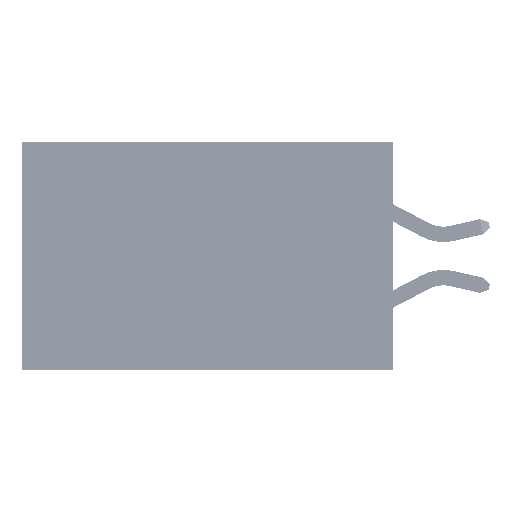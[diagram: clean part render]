
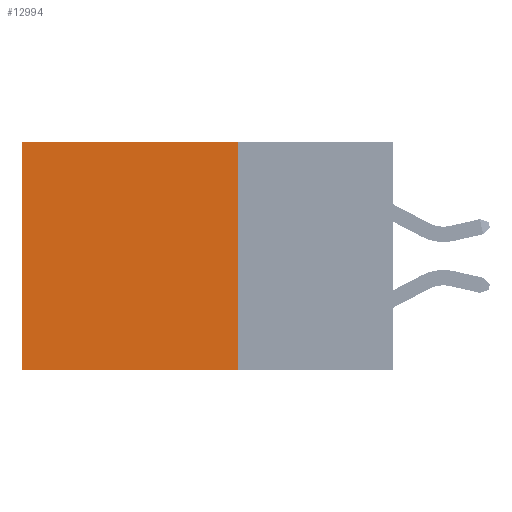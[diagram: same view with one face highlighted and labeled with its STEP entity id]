
A CAD part, left-side view. The second image highlights one B-rep face of the part: STEP entity #12994.
In plain terms, the highlighted planar face has unit normal (-1, 0, 0).
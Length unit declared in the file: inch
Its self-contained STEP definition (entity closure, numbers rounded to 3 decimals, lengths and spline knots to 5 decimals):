
#350 = DIRECTION ( 'NONE',  ( 0., 1., 0. ) ) ;
#1500 = DIRECTION ( 'NONE',  ( 0., 0., -1. ) ) ;
#3335 = ORIENTED_EDGE ( 'NONE', *, *, #19164, .F. ) ;
#4283 = LINE ( 'NONE', #19278, #27918 ) ;
#7785 = CARTESIAN_POINT ( 'NONE',  ( 0.2875, 0.6, -0.37 ) ) ;
#9209 = CARTESIAN_POINT ( 'NONE',  ( 0.2875, 0.25, 0. ) ) ;
#9853 = DIRECTION ( 'NONE',  ( 1., 0., 0. ) ) ;
#11382 = EDGE_LOOP ( 'NONE', ( #16281, #30564, #3335, #38147 ) ) ;
#12994 = ADVANCED_FACE ( 'NONE', ( #17235 ), #32239, .F. ) ;
#13551 = DIRECTION ( 'NONE',  ( 0., 0., -1. ) ) ;
#13638 = LINE ( 'NONE', #9209, #31500 ) ;
#15596 = VERTEX_POINT ( 'NONE', #26380 ) ;
#16281 = ORIENTED_EDGE ( 'NONE', *, *, #23016, .T. ) ;
#17235 = FACE_OUTER_BOUND ( 'NONE', #11382, .T. ) ;
#19063 = DIRECTION ( 'NONE',  ( 0., 0., -1. ) ) ;
#19164 = EDGE_CURVE ( 'NONE', #39890, #15596, #46018, .T. ) ;
#19278 = CARTESIAN_POINT ( 'NONE',  ( 0.2875, 0.25, -0.37 ) ) ;
#23016 = EDGE_CURVE ( 'NONE', #41914, #44384, #45142, .T. ) ;
#24217 = DIRECTION ( 'NONE',  ( 0., 1., 0. ) ) ;
#26380 = CARTESIAN_POINT ( 'NONE',  ( 0.2875, 0.25, -0.37 ) ) ;
#27918 = VECTOR ( 'NONE', #350, 39.37008 ) ;
#28887 = EDGE_CURVE ( 'NONE', #39890, #41914, #13638, .T. ) ;
#30564 = ORIENTED_EDGE ( 'NONE', *, *, #45771, .F. ) ;
#31500 = VECTOR ( 'NONE', #24217, 39.37008 ) ;
#32239 = PLANE ( 'NONE',  #46364 ) ;
#35933 = VECTOR ( 'NONE', #19063, 39.37008 ) ;
#38147 = ORIENTED_EDGE ( 'NONE', *, *, #28887, .T. ) ;
#38473 = CARTESIAN_POINT ( 'NONE',  ( 0.2875, 0.6, 0. ) ) ;
#39890 = VERTEX_POINT ( 'NONE', #41590 ) ;
#41590 = CARTESIAN_POINT ( 'NONE',  ( 0.2875, 0.25, 0. ) ) ;
#41914 = VERTEX_POINT ( 'NONE', #48236 ) ;
#42882 = VECTOR ( 'NONE', #1500, 39.37008 ) ;
#44384 = VERTEX_POINT ( 'NONE', #7785 ) ;
#45142 = LINE ( 'NONE', #38473, #35933 ) ;
#45771 = EDGE_CURVE ( 'NONE', #15596, #44384, #4283, .T. ) ;
#46018 = LINE ( 'NONE', #46748, #42882 ) ;
#46364 = AXIS2_PLACEMENT_3D ( 'NONE', #47243, #9853, #13551 ) ;
#46748 = CARTESIAN_POINT ( 'NONE',  ( 0.2875, 0.25, 0. ) ) ;
#47243 = CARTESIAN_POINT ( 'NONE',  ( 0.2875, 0.25, 0. ) ) ;
#48236 = CARTESIAN_POINT ( 'NONE',  ( 0.2875, 0.6, 0. ) ) ;
